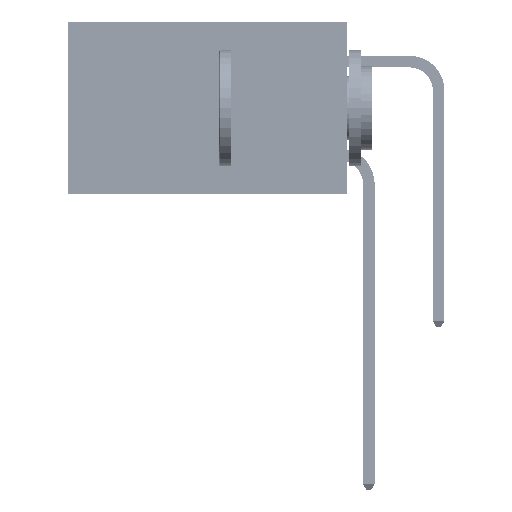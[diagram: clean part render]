
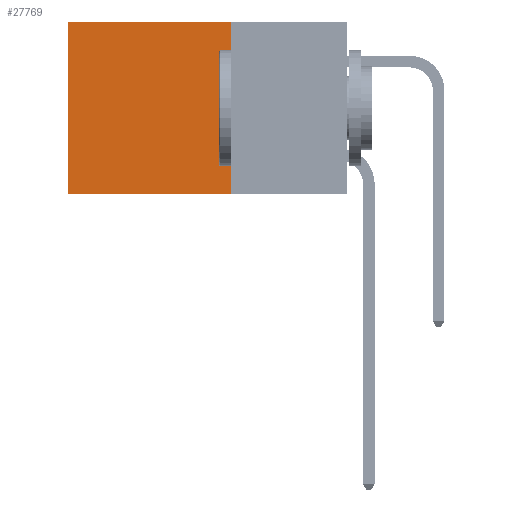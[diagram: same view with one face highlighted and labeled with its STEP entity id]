
A CAD part, left-side view. The second image highlights one B-rep face of the part: STEP entity #27769.
In plain terms, the highlighted planar face has unit normal (-1, 0, 0).
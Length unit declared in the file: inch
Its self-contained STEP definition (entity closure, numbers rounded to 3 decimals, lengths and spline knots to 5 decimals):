
#1156 = EDGE_CURVE ( 'NONE', #31024, #31127, #2731, .T. ) ;
#2607 = CARTESIAN_POINT ( 'NONE',  ( 0.2875, 0.25, 0. ) ) ;
#2731 = LINE ( 'NONE', #33074, #21028 ) ;
#3664 = ORIENTED_EDGE ( 'NONE', *, *, #20148, .T. ) ;
#3818 = ORIENTED_EDGE ( 'NONE', *, *, #18368, .F. ) ;
#7501 = LINE ( 'NONE', #30462, #43771 ) ;
#7605 = DIRECTION ( 'NONE',  ( 0., 1., 0. ) ) ;
#9679 = CARTESIAN_POINT ( 'NONE',  ( 0.2875, 0.6, -0.37 ) ) ;
#10932 = DIRECTION ( 'NONE',  ( 0., 0., -1. ) ) ;
#11513 = CARTESIAN_POINT ( 'NONE',  ( 0.2875, 0.25, -0.37 ) ) ;
#12319 = DIRECTION ( 'NONE',  ( 0., 0., -1. ) ) ;
#15200 = DIRECTION ( 'NONE',  ( 0., 1., 0. ) ) ;
#17901 = CARTESIAN_POINT ( 'NONE',  ( 0.2875, 0.6, 0. ) ) ;
#18368 = EDGE_CURVE ( 'NONE', #31024, #22471, #7501, .T. ) ;
#20148 = EDGE_CURVE ( 'NONE', #31127, #43409, #25584, .T. ) ;
#21028 = VECTOR ( 'NONE', #7605, 39.37008 ) ;
#22471 = VERTEX_POINT ( 'NONE', #41461 ) ;
#23023 = ORIENTED_EDGE ( 'NONE', *, *, #1156, .T. ) ;
#23237 = FACE_OUTER_BOUND ( 'NONE', #28387, .T. ) ;
#25459 = CARTESIAN_POINT ( 'NONE',  ( 0.2875, 0.25, 0. ) ) ;
#25584 = LINE ( 'NONE', #17901, #35206 ) ;
#26083 = EDGE_CURVE ( 'NONE', #22471, #43409, #27377, .T. ) ;
#27377 = LINE ( 'NONE', #11513, #45381 ) ;
#27769 = ADVANCED_FACE ( 'NONE', ( #23237 ), #29097, .F. ) ;
#28387 = EDGE_LOOP ( 'NONE', ( #3664, #37091, #3818, #23023 ) ) ;
#29097 = PLANE ( 'NONE',  #38580 ) ;
#30462 = CARTESIAN_POINT ( 'NONE',  ( 0.2875, 0.25, 0. ) ) ;
#31024 = VERTEX_POINT ( 'NONE', #2607 ) ;
#31127 = VERTEX_POINT ( 'NONE', #39439 ) ;
#32749 = DIRECTION ( 'NONE',  ( 1., 0., 0. ) ) ;
#33074 = CARTESIAN_POINT ( 'NONE',  ( 0.2875, 0.25, 0. ) ) ;
#35206 = VECTOR ( 'NONE', #43169, 39.37008 ) ;
#37091 = ORIENTED_EDGE ( 'NONE', *, *, #26083, .F. ) ;
#38580 = AXIS2_PLACEMENT_3D ( 'NONE', #25459, #32749, #10932 ) ;
#39439 = CARTESIAN_POINT ( 'NONE',  ( 0.2875, 0.6, 0. ) ) ;
#41461 = CARTESIAN_POINT ( 'NONE',  ( 0.2875, 0.25, -0.37 ) ) ;
#43169 = DIRECTION ( 'NONE',  ( 0., 0., -1. ) ) ;
#43409 = VERTEX_POINT ( 'NONE', #9679 ) ;
#43771 = VECTOR ( 'NONE', #12319, 39.37008 ) ;
#45381 = VECTOR ( 'NONE', #15200, 39.37008 ) ;
